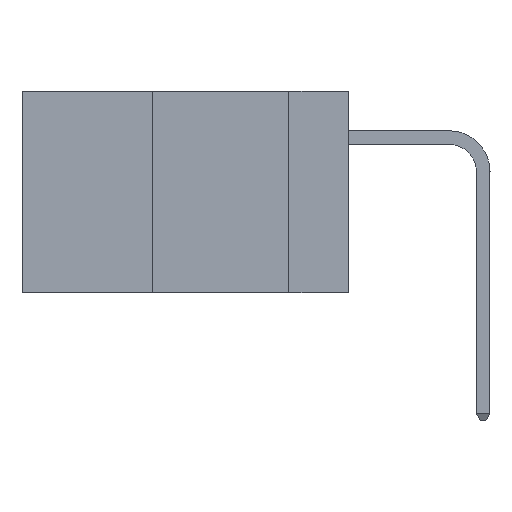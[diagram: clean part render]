
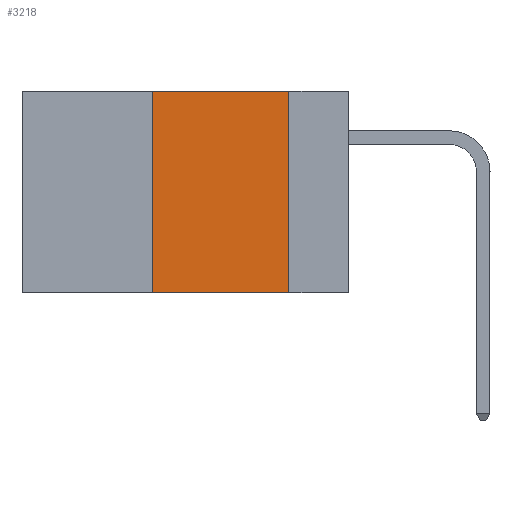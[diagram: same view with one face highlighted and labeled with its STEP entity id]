
A CAD part, left-side view. The second image highlights one B-rep face of the part: STEP entity #3218.
In plain terms, the highlighted planar face has unit normal (-1, 0, 0).
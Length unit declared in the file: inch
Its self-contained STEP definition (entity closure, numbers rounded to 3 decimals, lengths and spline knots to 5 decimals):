
#613 = DIRECTION ( 'NONE',  ( 0., 0., 1. ) ) ;
#693 = CARTESIAN_POINT ( 'NONE',  ( 0., 0.11, 0. ) ) ;
#1250 = VERTEX_POINT ( 'NONE', #12387 ) ;
#1284 = EDGE_CURVE ( 'NONE', #12121, #15177, #16148, .T. ) ;
#1683 = CARTESIAN_POINT ( 'NONE',  ( 0., 0.11, -0.37 ) ) ;
#1807 = FACE_OUTER_BOUND ( 'NONE', #14262, .T. ) ;
#1834 = AXIS2_PLACEMENT_3D ( 'NONE', #5484, #11485, #13028 ) ;
#2092 = EDGE_CURVE ( 'NONE', #12121, #15009, #5367, .T. ) ;
#2147 = EDGE_CURVE ( 'NONE', #15177, #1250, #14802, .T. ) ;
#2564 = ORIENTED_EDGE ( 'NONE', *, *, #1284, .F. ) ;
#2974 = VECTOR ( 'NONE', #16114, 39.37008 ) ;
#3149 = DIRECTION ( 'NONE',  ( 0., 0., -1. ) ) ;
#3218 = ADVANCED_FACE ( 'NONE', ( #1807 ), #6458, .F. ) ;
#3423 = CARTESIAN_POINT ( 'NONE',  ( 0., 0.6, 0. ) ) ;
#3650 = CARTESIAN_POINT ( 'NONE',  ( 0., 0.36, -0.37 ) ) ;
#4275 = VECTOR ( 'NONE', #14150, 39.37008 ) ;
#5367 = LINE ( 'NONE', #13092, #4275 ) ;
#5484 = CARTESIAN_POINT ( 'NONE',  ( 0., 0.6, 0. ) ) ;
#6458 = PLANE ( 'NONE',  #1834 ) ;
#7225 = LINE ( 'NONE', #693, #7471 ) ;
#7471 = VECTOR ( 'NONE', #3149, 39.37008 ) ;
#8307 = VECTOR ( 'NONE', #613, 39.37008 ) ;
#9763 = EDGE_CURVE ( 'NONE', #1250, #15009, #7225, .T. ) ;
#11485 = DIRECTION ( 'NONE',  ( 1., 0., 0. ) ) ;
#11889 = ORIENTED_EDGE ( 'NONE', *, *, #9763, .F. ) ;
#12121 = VERTEX_POINT ( 'NONE', #3650 ) ;
#12387 = CARTESIAN_POINT ( 'NONE',  ( 0., 0.11, 0. ) ) ;
#12410 = CARTESIAN_POINT ( 'NONE',  ( 0., 0.36, 0. ) ) ;
#12414 = ORIENTED_EDGE ( 'NONE', *, *, #2147, .F. ) ;
#13028 = DIRECTION ( 'NONE',  ( 0., 0., -1. ) ) ;
#13092 = CARTESIAN_POINT ( 'NONE',  ( 0., 0.6, -0.37 ) ) ;
#13118 = ORIENTED_EDGE ( 'NONE', *, *, #2092, .T. ) ;
#13312 = CARTESIAN_POINT ( 'NONE',  ( 0., 0.36, 0. ) ) ;
#14150 = DIRECTION ( 'NONE',  ( 0., -1., 0. ) ) ;
#14262 = EDGE_LOOP ( 'NONE', ( #11889, #12414, #2564, #13118 ) ) ;
#14802 = LINE ( 'NONE', #3423, #2974 ) ;
#15009 = VERTEX_POINT ( 'NONE', #1683 ) ;
#15177 = VERTEX_POINT ( 'NONE', #12410 ) ;
#16114 = DIRECTION ( 'NONE',  ( 0., -1., 0. ) ) ;
#16148 = LINE ( 'NONE', #13312, #8307 ) ;
